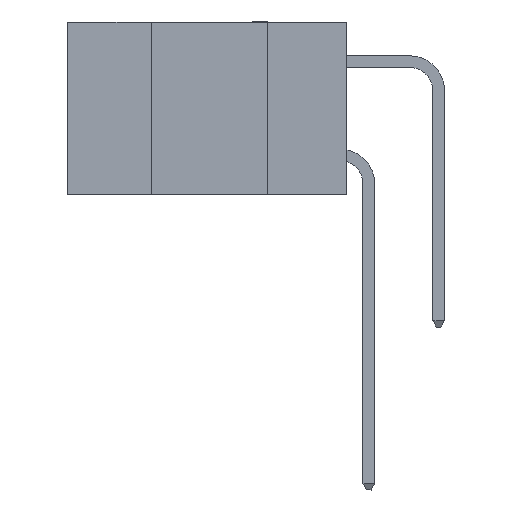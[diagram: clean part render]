
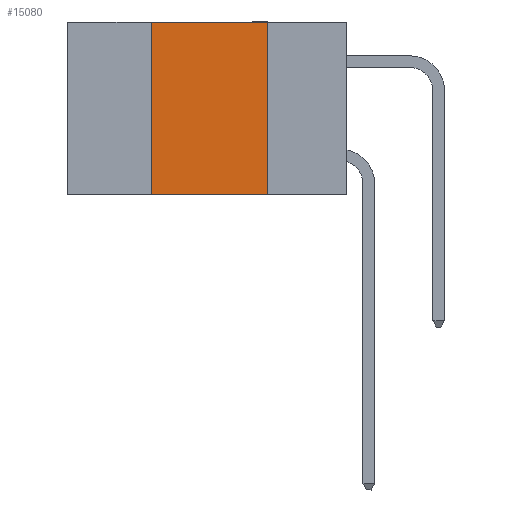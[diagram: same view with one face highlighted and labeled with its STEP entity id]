
A CAD part, left-side view. The second image highlights one B-rep face of the part: STEP entity #15080.
In plain terms, the highlighted planar face has unit normal (-1, 0, 0).
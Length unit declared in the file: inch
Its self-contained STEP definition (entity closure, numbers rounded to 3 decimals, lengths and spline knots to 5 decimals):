
#255 = CARTESIAN_POINT ( 'NONE',  ( 0., 0.17, 0. ) ) ;
#1166 = ORIENTED_EDGE ( 'NONE', *, *, #2520, .F. ) ;
#1504 = CARTESIAN_POINT ( 'NONE',  ( 0., 0.42, -0.37 ) ) ;
#2320 = DIRECTION ( 'NONE',  ( 0., -1., 0. ) ) ;
#2520 = EDGE_CURVE ( 'NONE', #5842, #5520, #19419, .T. ) ;
#3199 = FACE_OUTER_BOUND ( 'NONE', #8854, .T. ) ;
#4153 = LINE ( 'NONE', #6600, #25132 ) ;
#4750 = VECTOR ( 'NONE', #5663, 39.37008 ) ;
#4931 = VECTOR ( 'NONE', #8241, 39.37008 ) ;
#5520 = VERTEX_POINT ( 'NONE', #24202 ) ;
#5540 = EDGE_CURVE ( 'NONE', #11212, #11102, #12222, .T. ) ;
#5622 = AXIS2_PLACEMENT_3D ( 'NONE', #16704, #18377, #24582 ) ;
#5663 = DIRECTION ( 'NONE',  ( 0., 0., 1. ) ) ;
#5842 = VERTEX_POINT ( 'NONE', #1504 ) ;
#6600 = CARTESIAN_POINT ( 'NONE',  ( 0., 0.6, -0.37 ) ) ;
#7182 = PLANE ( 'NONE',  #5622 ) ;
#8241 = DIRECTION ( 'NONE',  ( 0., 0., -1. ) ) ;
#8854 = EDGE_LOOP ( 'NONE', ( #25088, #17920, #1166, #14765 ) ) ;
#9540 = EDGE_CURVE ( 'NONE', #5520, #11212, #24091, .T. ) ;
#10102 = VECTOR ( 'NONE', #2320, 39.37008 ) ;
#10344 = DIRECTION ( 'NONE',  ( 0., -1., 0. ) ) ;
#11102 = VERTEX_POINT ( 'NONE', #16354 ) ;
#11212 = VERTEX_POINT ( 'NONE', #17230 ) ;
#12222 = LINE ( 'NONE', #255, #4931 ) ;
#14765 = ORIENTED_EDGE ( 'NONE', *, *, #19645, .T. ) ;
#15080 = ADVANCED_FACE ( 'NONE', ( #3199 ), #7182, .F. ) ;
#16354 = CARTESIAN_POINT ( 'NONE',  ( 0., 0.17, -0.37 ) ) ;
#16704 = CARTESIAN_POINT ( 'NONE',  ( 0., 0.6, 0. ) ) ;
#17230 = CARTESIAN_POINT ( 'NONE',  ( 0., 0.17, 0. ) ) ;
#17920 = ORIENTED_EDGE ( 'NONE', *, *, #9540, .F. ) ;
#18377 = DIRECTION ( 'NONE',  ( 1., 0., 0. ) ) ;
#19419 = LINE ( 'NONE', #21497, #4750 ) ;
#19571 = CARTESIAN_POINT ( 'NONE',  ( 0., 0.6, 0. ) ) ;
#19645 = EDGE_CURVE ( 'NONE', #5842, #11102, #4153, .T. ) ;
#21497 = CARTESIAN_POINT ( 'NONE',  ( 0., 0.42, 0. ) ) ;
#24091 = LINE ( 'NONE', #19571, #10102 ) ;
#24202 = CARTESIAN_POINT ( 'NONE',  ( 0., 0.42, 0. ) ) ;
#24582 = DIRECTION ( 'NONE',  ( 0., 0., -1. ) ) ;
#25088 = ORIENTED_EDGE ( 'NONE', *, *, #5540, .F. ) ;
#25132 = VECTOR ( 'NONE', #10344, 39.37008 ) ;
